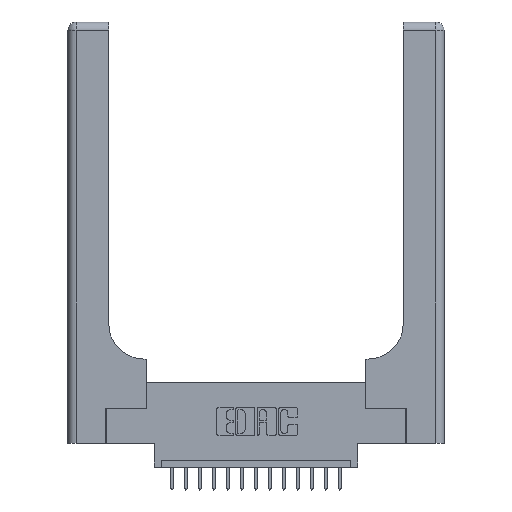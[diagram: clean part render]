
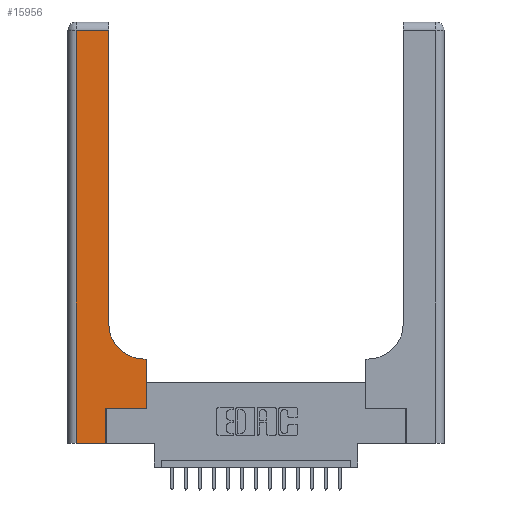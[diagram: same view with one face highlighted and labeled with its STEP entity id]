
A CAD part, top view. The second image highlights one B-rep face of the part: STEP entity #15956.
In plain terms, the highlighted planar face has unit normal (0, 0, 1).
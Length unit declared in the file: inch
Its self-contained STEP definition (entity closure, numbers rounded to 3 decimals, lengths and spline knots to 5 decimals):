
#746 = VECTOR ( 'NONE', #9653, 39.37008 ) ;
#1152 = ORIENTED_EDGE ( 'NONE', *, *, #12544, .T. ) ;
#1280 = DIRECTION ( 'NONE',  ( -1., 0., 0. ) ) ;
#1550 = CARTESIAN_POINT ( 'NONE',  ( 0., 3., 0.37 ) ) ;
#1809 = PLANE ( 'NONE',  #4070 ) ;
#1930 = DIRECTION ( 'NONE',  ( 0., 0., -1. ) ) ;
#1992 = DIRECTION ( 'NONE',  ( 1., 0., 0. ) ) ;
#2017 = VERTEX_POINT ( 'NONE', #12700 ) ;
#2362 = CARTESIAN_POINT ( 'NONE',  ( 0., 0., 0.37 ) ) ;
#3027 = CARTESIAN_POINT ( 'NONE',  ( 0.5415, 0.6, 0.37 ) ) ;
#3296 = VERTEX_POINT ( 'NONE', #14509 ) ;
#3547 = EDGE_CURVE ( 'NONE', #11318, #10446, #5633, .T. ) ;
#3737 = DIRECTION ( 'NONE',  ( 0., 1., 0. ) ) ;
#3845 = ORIENTED_EDGE ( 'NONE', *, *, #11827, .T. ) ;
#4070 = AXIS2_PLACEMENT_3D ( 'NONE', #1550, #17756, #8896 ) ;
#4266 = CARTESIAN_POINT ( 'NONE',  ( 0.06, 3., 0.37 ) ) ;
#4398 = ORIENTED_EDGE ( 'NONE', *, *, #14204, .T. ) ;
#4484 = VECTOR ( 'NONE', #13540, 39.37008 ) ;
#4487 = EDGE_CURVE ( 'NONE', #3296, #13837, #17857, .T. ) ;
#5186 = LINE ( 'NONE', #4266, #9781 ) ;
#5537 = EDGE_CURVE ( 'NONE', #16594, #3296, #8990, .T. ) ;
#5633 = LINE ( 'NONE', #10640, #4484 ) ;
#5671 = CARTESIAN_POINT ( 'NONE',  ( 0.5585, 0.25, 0.37 ) ) ;
#6385 = VECTOR ( 'NONE', #1280, 39.37008 ) ;
#6614 = VECTOR ( 'NONE', #17191, 39.37008 ) ;
#6801 = DIRECTION ( 'NONE',  ( 1., 0., 0. ) ) ;
#7305 = VERTEX_POINT ( 'NONE', #16176 ) ;
#7541 = ORIENTED_EDGE ( 'NONE', *, *, #14941, .T. ) ;
#8353 = EDGE_LOOP ( 'NONE', ( #12076, #3845, #4398, #10178, #8491, #1152, #17524, #17891, #7541 ) ) ;
#8485 = CARTESIAN_POINT ( 'NONE',  ( 0.269, 0.25, 0.37 ) ) ;
#8491 = ORIENTED_EDGE ( 'NONE', *, *, #15223, .T. ) ;
#8769 = DIRECTION ( 'NONE',  ( 0., -1., 0. ) ) ;
#8896 = DIRECTION ( 'NONE',  ( -1., 0., 0. ) ) ;
#8957 = CARTESIAN_POINT ( 'NONE',  ( 0.2915, 0.6, 0.37 ) ) ;
#8990 = LINE ( 'NONE', #9767, #746 ) ;
#9653 = DIRECTION ( 'NONE',  ( 0., 1., 0. ) ) ;
#9739 = AXIS2_PLACEMENT_3D ( 'NONE', #13622, #1930, #1992 ) ;
#9767 = CARTESIAN_POINT ( 'NONE',  ( 0.5585, 0.25, 0.37 ) ) ;
#9781 = VECTOR ( 'NONE', #8769, 39.37008 ) ;
#9991 = VECTOR ( 'NONE', #18209, 39.37008 ) ;
#10178 = ORIENTED_EDGE ( 'NONE', *, *, #18709, .T. ) ;
#10446 = VERTEX_POINT ( 'NONE', #18784 ) ;
#10640 = CARTESIAN_POINT ( 'NONE',  ( 0.2915, 3., 0.37 ) ) ;
#11259 = CARTESIAN_POINT ( 'NONE',  ( 0.269, 0., 0.37 ) ) ;
#11318 = VERTEX_POINT ( 'NONE', #16347 ) ;
#11364 = LINE ( 'NONE', #11259, #16902 ) ;
#11474 = LINE ( 'NONE', #14398, #6385 ) ;
#11744 = CARTESIAN_POINT ( 'NONE',  ( 0.269, 0., 0.37 ) ) ;
#11827 = EDGE_CURVE ( 'NONE', #10446, #7305, #11474, .T. ) ;
#12076 = ORIENTED_EDGE ( 'NONE', *, *, #3547, .T. ) ;
#12544 = EDGE_CURVE ( 'NONE', #16971, #16594, #18853, .T. ) ;
#12700 = CARTESIAN_POINT ( 'NONE',  ( 0.06, 0., 0.37 ) ) ;
#13099 = LINE ( 'NONE', #2362, #6614 ) ;
#13540 = DIRECTION ( 'NONE',  ( 0., 1., 0. ) ) ;
#13622 = CARTESIAN_POINT ( 'NONE',  ( 0.5415, 0.85, 0.37 ) ) ;
#13794 = VERTEX_POINT ( 'NONE', #11744 ) ;
#13837 = VERTEX_POINT ( 'NONE', #3027 ) ;
#13944 = CIRCLE ( 'NONE', #9739, 0.25 ) ;
#14204 = EDGE_CURVE ( 'NONE', #7305, #2017, #5186, .T. ) ;
#14398 = CARTESIAN_POINT ( 'NONE',  ( 0., 2.94, 0.37 ) ) ;
#14509 = CARTESIAN_POINT ( 'NONE',  ( 0.5585, 0.6, 0.37 ) ) ;
#14941 = EDGE_CURVE ( 'NONE', #13837, #11318, #13944, .T. ) ;
#15223 = EDGE_CURVE ( 'NONE', #13794, #16971, #11364, .T. ) ;
#15956 = ADVANCED_FACE ( 'NONE', ( #15958 ), #1809, .F. ) ;
#15958 = FACE_OUTER_BOUND ( 'NONE', #8353, .T. ) ;
#16062 = VECTOR ( 'NONE', #6801, 39.37008 ) ;
#16176 = CARTESIAN_POINT ( 'NONE',  ( 0.06, 2.94, 0.37 ) ) ;
#16347 = CARTESIAN_POINT ( 'NONE',  ( 0.2915, 0.85, 0.37 ) ) ;
#16594 = VERTEX_POINT ( 'NONE', #5671 ) ;
#16902 = VECTOR ( 'NONE', #3737, 39.37008 ) ;
#16971 = VERTEX_POINT ( 'NONE', #8485 ) ;
#17191 = DIRECTION ( 'NONE',  ( 1., 0., 0. ) ) ;
#17524 = ORIENTED_EDGE ( 'NONE', *, *, #5537, .T. ) ;
#17756 = DIRECTION ( 'NONE',  ( 0., 0., -1. ) ) ;
#17857 = LINE ( 'NONE', #8957, #9991 ) ;
#17891 = ORIENTED_EDGE ( 'NONE', *, *, #4487, .T. ) ;
#18209 = DIRECTION ( 'NONE',  ( -1., 0., 0. ) ) ;
#18709 = EDGE_CURVE ( 'NONE', #2017, #13794, #13099, .T. ) ;
#18759 = CARTESIAN_POINT ( 'NONE',  ( 0.269, 0.25, 0.37 ) ) ;
#18784 = CARTESIAN_POINT ( 'NONE',  ( 0.2915, 2.94, 0.37 ) ) ;
#18853 = LINE ( 'NONE', #18759, #16062 ) ;
